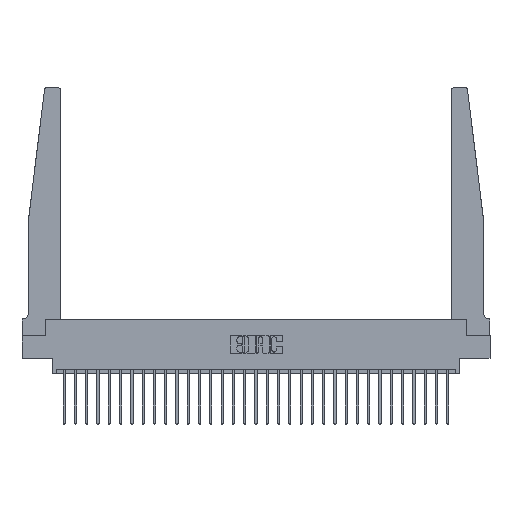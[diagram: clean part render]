
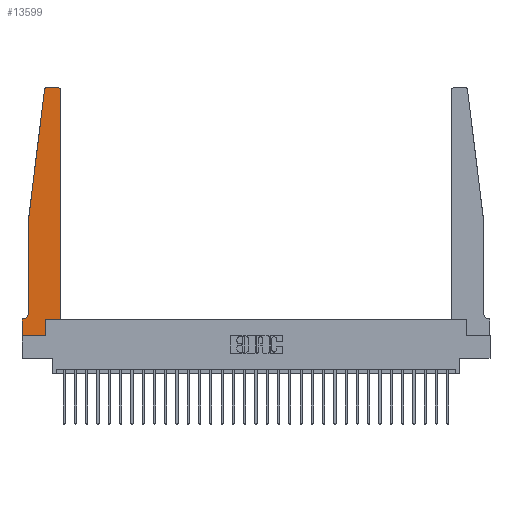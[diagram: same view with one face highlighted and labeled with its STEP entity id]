
A CAD part, top view. The second image highlights one B-rep face of the part: STEP entity #13599.
In plain terms, the highlighted planar face has unit normal (0, 0, 1).
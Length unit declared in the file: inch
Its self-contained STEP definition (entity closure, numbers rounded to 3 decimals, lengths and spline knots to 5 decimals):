
#290 = ORIENTED_EDGE ( 'NONE', *, *, #24238, .T. ) ;
#732 = LINE ( 'NONE', #2935, #28984 ) ;
#1095 = CARTESIAN_POINT ( 'NONE',  ( 0.065, 0.2375, 0.37 ) ) ;
#1133 = VERTEX_POINT ( 'NONE', #24853 ) ;
#1362 = CIRCLE ( 'NONE', #24430, 0.03 ) ;
#1484 = VERTEX_POINT ( 'NONE', #17154 ) ;
#1552 = CARTESIAN_POINT ( 'NONE',  ( 0.425, 0.18, 0.37 ) ) ;
#1900 = EDGE_CURVE ( 'NONE', #1484, #5035, #1362, .T. ) ;
#2198 = DIRECTION ( 'NONE',  ( -1., 0., 0. ) ) ;
#2355 = VERTEX_POINT ( 'NONE', #26786 ) ;
#2493 = LINE ( 'NONE', #4715, #9287 ) ;
#2935 = CARTESIAN_POINT ( 'NONE',  ( 0.065, 1.25, 0.37 ) ) ;
#3225 = PLANE ( 'NONE',  #16817 ) ;
#3534 = VECTOR ( 'NONE', #11213, 39.37008 ) ;
#3665 = DIRECTION ( 'NONE',  ( 0., 1., 0. ) ) ;
#3712 = EDGE_CURVE ( 'NONE', #17471, #23856, #6325, .T. ) ;
#4280 = DIRECTION ( 'NONE',  ( 1., 0., 0. ) ) ;
#4581 = VERTEX_POINT ( 'NONE', #22671 ) ;
#4715 = CARTESIAN_POINT ( 'NONE',  ( 0., 0., 0.37 ) ) ;
#4764 = CARTESIAN_POINT ( 'NONE',  ( 0.015, 0.2375, 0.37 ) ) ;
#4936 = LINE ( 'NONE', #25419, #22850 ) ;
#5035 = VERTEX_POINT ( 'NONE', #18235 ) ;
#5870 = ORIENTED_EDGE ( 'NONE', *, *, #3712, .T. ) ;
#6026 = AXIS2_PLACEMENT_3D ( 'NONE', #4764, #15506, #19933 ) ;
#6217 = VECTOR ( 'NONE', #28947, 39.37008 ) ;
#6325 = LINE ( 'NONE', #26675, #13675 ) ;
#6861 = VECTOR ( 'NONE', #18916, 39.37008 ) ;
#8799 = CARTESIAN_POINT ( 'NONE',  ( 0.425, 0.18, 0.37 ) ) ;
#8874 = LINE ( 'NONE', #15193, #6217 ) ;
#9287 = VECTOR ( 'NONE', #24604, 39.37008 ) ;
#9898 = VERTEX_POINT ( 'NONE', #1095 ) ;
#10018 = DIRECTION ( 'NONE',  ( 0., 0., 1. ) ) ;
#10368 = EDGE_CURVE ( 'NONE', #2355, #25717, #25303, .T. ) ;
#10911 = CARTESIAN_POINT ( 'NONE',  ( 0.27653, 2.72, 0.37 ) ) ;
#11213 = DIRECTION ( 'NONE',  ( -1., 0., 0. ) ) ;
#11234 = EDGE_CURVE ( 'NONE', #23856, #20172, #4936, .T. ) ;
#12817 = EDGE_CURVE ( 'NONE', #9898, #17282, #15886, .T. ) ;
#12902 = VECTOR ( 'NONE', #25341, 39.37008 ) ;
#13057 = ORIENTED_EDGE ( 'NONE', *, *, #1900, .T. ) ;
#13182 = VERTEX_POINT ( 'NONE', #21245 ) ;
#13267 = ORIENTED_EDGE ( 'NONE', *, *, #10368, .T. ) ;
#13599 = ADVANCED_FACE ( 'NONE', ( #19280 ), #3225, .T. ) ;
#13675 = VECTOR ( 'NONE', #3665, 39.37008 ) ;
#13996 = LINE ( 'NONE', #20057, #3534 ) ;
#14393 = EDGE_CURVE ( 'NONE', #17282, #13182, #18114, .T. ) ;
#14497 = EDGE_CURVE ( 'NONE', #20172, #2355, #27585, .T. ) ;
#14869 = EDGE_CURVE ( 'NONE', #4581, #9898, #26138, .T. ) ;
#14997 = CARTESIAN_POINT ( 'NONE',  ( 0.015, 0.1875, 0.37 ) ) ;
#15193 = CARTESIAN_POINT ( 'NONE',  ( 0., 0., 0.37 ) ) ;
#15218 = ORIENTED_EDGE ( 'NONE', *, *, #26037, .T. ) ;
#15465 = CARTESIAN_POINT ( 'NONE',  ( 0.395, 2.75, 0.37 ) ) ;
#15506 = DIRECTION ( 'NONE',  ( 0., 0., -1. ) ) ;
#15593 = CARTESIAN_POINT ( 'NONE',  ( 0.065, 0.1875, 0.37 ) ) ;
#15640 = EDGE_CURVE ( 'NONE', #1133, #17471, #2493, .T. ) ;
#15801 = ORIENTED_EDGE ( 'NONE', *, *, #11234, .T. ) ;
#15886 = CIRCLE ( 'NONE', #6026, 0.05 ) ;
#16817 = AXIS2_PLACEMENT_3D ( 'NONE', #28315, #10018, #17077 ) ;
#17037 = EDGE_LOOP ( 'NONE', ( #290, #13057, #15218, #22775, #23536, #26922, #17894, #27684, #5870, #15801, #25026, #13267 ) ) ;
#17077 = DIRECTION ( 'NONE',  ( 1., 0., 0. ) ) ;
#17154 = CARTESIAN_POINT ( 'NONE',  ( 0.27653, 2.75, 0.37 ) ) ;
#17282 = VERTEX_POINT ( 'NONE', #14997 ) ;
#17471 = VERTEX_POINT ( 'NONE', #17813 ) ;
#17813 = CARTESIAN_POINT ( 'NONE',  ( 0.2605, 0., 0.37 ) ) ;
#17894 = ORIENTED_EDGE ( 'NONE', *, *, #21052, .T. ) ;
#18114 = LINE ( 'NONE', #15593, #27058 ) ;
#18235 = CARTESIAN_POINT ( 'NONE',  ( 0.24675, 2.72367, 0.37 ) ) ;
#18916 = DIRECTION ( 'NONE',  ( 0., -1., 0. ) ) ;
#19181 = AXIS2_PLACEMENT_3D ( 'NONE', #28233, #21407, #26295 ) ;
#19280 = FACE_OUTER_BOUND ( 'NONE', #17037, .T. ) ;
#19933 = DIRECTION ( 'NONE',  ( -1., 0., 0. ) ) ;
#20036 = DIRECTION ( 'NONE',  ( 0., 0., 1. ) ) ;
#20057 = CARTESIAN_POINT ( 'NONE',  ( 0.25, 2.75, 0.37 ) ) ;
#20172 = VERTEX_POINT ( 'NONE', #8799 ) ;
#20701 = DIRECTION ( 'NONE',  ( 1., 0., 0. ) ) ;
#21052 = EDGE_CURVE ( 'NONE', #13182, #1133, #8874, .T. ) ;
#21245 = CARTESIAN_POINT ( 'NONE',  ( 0., 0.1875, 0.37 ) ) ;
#21407 = DIRECTION ( 'NONE',  ( 0., 0., 1. ) ) ;
#22671 = CARTESIAN_POINT ( 'NONE',  ( 0.065, 1.25, 0.37 ) ) ;
#22775 = ORIENTED_EDGE ( 'NONE', *, *, #14869, .T. ) ;
#22850 = VECTOR ( 'NONE', #20701, 39.37008 ) ;
#23479 = CARTESIAN_POINT ( 'NONE',  ( 0.065, 1.25, 0.37 ) ) ;
#23536 = ORIENTED_EDGE ( 'NONE', *, *, #12817, .T. ) ;
#23582 = DIRECTION ( 'NONE',  ( -0.122, -0.992, 0. ) ) ;
#23856 = VERTEX_POINT ( 'NONE', #25986 ) ;
#24238 = EDGE_CURVE ( 'NONE', #25717, #1484, #13996, .T. ) ;
#24430 = AXIS2_PLACEMENT_3D ( 'NONE', #10911, #20036, #4280 ) ;
#24604 = DIRECTION ( 'NONE',  ( 1., 0., 0. ) ) ;
#24853 = CARTESIAN_POINT ( 'NONE',  ( 0., 0., 0.37 ) ) ;
#25026 = ORIENTED_EDGE ( 'NONE', *, *, #14497, .T. ) ;
#25303 = CIRCLE ( 'NONE', #19181, 0.03 ) ;
#25341 = DIRECTION ( 'NONE',  ( 0., 1., 0. ) ) ;
#25419 = CARTESIAN_POINT ( 'NONE',  ( 0.425, 0.18, 0.37 ) ) ;
#25717 = VERTEX_POINT ( 'NONE', #15465 ) ;
#25986 = CARTESIAN_POINT ( 'NONE',  ( 0.2605, 0.18, 0.37 ) ) ;
#26037 = EDGE_CURVE ( 'NONE', #5035, #4581, #732, .T. ) ;
#26138 = LINE ( 'NONE', #23479, #6861 ) ;
#26295 = DIRECTION ( 'NONE',  ( 1., 0., 0. ) ) ;
#26675 = CARTESIAN_POINT ( 'NONE',  ( 0.2605, 0.18, 0.37 ) ) ;
#26786 = CARTESIAN_POINT ( 'NONE',  ( 0.425, 2.72, 0.37 ) ) ;
#26922 = ORIENTED_EDGE ( 'NONE', *, *, #14393, .T. ) ;
#27058 = VECTOR ( 'NONE', #2198, 39.37008 ) ;
#27585 = LINE ( 'NONE', #1552, #12902 ) ;
#27684 = ORIENTED_EDGE ( 'NONE', *, *, #15640, .T. ) ;
#28233 = CARTESIAN_POINT ( 'NONE',  ( 0.395, 2.72, 0.37 ) ) ;
#28315 = CARTESIAN_POINT ( 'NONE',  ( 0., 0.1875, 0.37 ) ) ;
#28947 = DIRECTION ( 'NONE',  ( 0., -1., 0. ) ) ;
#28984 = VECTOR ( 'NONE', #23582, 39.37008 ) ;
